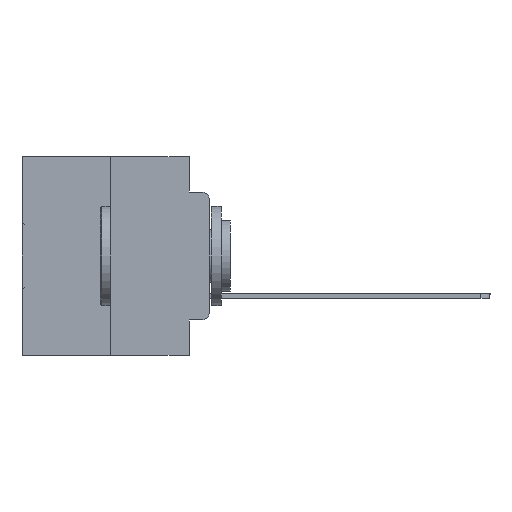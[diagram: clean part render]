
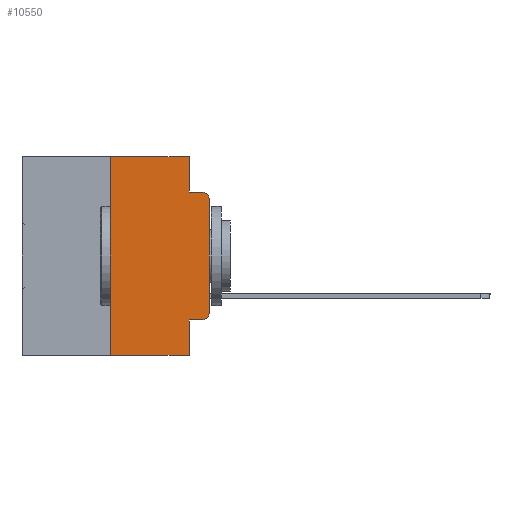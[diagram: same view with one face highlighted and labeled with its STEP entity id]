
A CAD part, left-side view. The second image highlights one B-rep face of the part: STEP entity #10550.
In plain terms, the highlighted planar face has unit normal (-1, 0, 0).
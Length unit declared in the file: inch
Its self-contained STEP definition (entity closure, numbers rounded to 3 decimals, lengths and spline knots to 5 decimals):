
#16 = ORIENTED_EDGE ( 'NONE', *, *, #12953, .T. ) ;
#106 = CARTESIAN_POINT ( 'NONE',  ( 0., 0.051, -0.4115 ) ) ;
#396 = CIRCLE ( 'NONE', #18454, 0.02 ) ;
#503 = CARTESIAN_POINT ( 'NONE',  ( 0., 0.25, 0. ) ) ;
#875 = PLANE ( 'NONE',  #8040 ) ;
#1307 = CARTESIAN_POINT ( 'NONE',  ( 0., 0.02, -0.3915 ) ) ;
#1934 = VECTOR ( 'NONE', #31414, 39.37008 ) ;
#2017 = CARTESIAN_POINT ( 'NONE',  ( 0., 0., -0.3915 ) ) ;
#2045 = DIRECTION ( 'NONE',  ( 0., -1., 0. ) ) ;
#3313 = VERTEX_POINT ( 'NONE', #2017 ) ;
#4301 = LINE ( 'NONE', #26386, #26181 ) ;
#4407 = EDGE_LOOP ( 'NONE', ( #9631, #14332, #9688, #22419, #19656, #26103, #17571, #27976, #16, #5335 ) ) ;
#4494 = VECTOR ( 'NONE', #8327, 39.37008 ) ;
#5335 = ORIENTED_EDGE ( 'NONE', *, *, #7993, .T. ) ;
#6140 = CARTESIAN_POINT ( 'NONE',  ( 0., 0.051, -0.5 ) ) ;
#6204 = CIRCLE ( 'NONE', #24243, 0.02 ) ;
#6547 = CARTESIAN_POINT ( 'NONE',  ( 0., 0.473, 0. ) ) ;
#6802 = VERTEX_POINT ( 'NONE', #503 ) ;
#6828 = CARTESIAN_POINT ( 'NONE',  ( 0., 0.25, -0.5 ) ) ;
#6910 = LINE ( 'NONE', #16754, #1934 ) ;
#7903 = VERTEX_POINT ( 'NONE', #20375 ) ;
#7993 = EDGE_CURVE ( 'NONE', #28216, #3313, #6204, .T. ) ;
#8040 = AXIS2_PLACEMENT_3D ( 'NONE', #6547, #10747, #25894 ) ;
#8327 = DIRECTION ( 'NONE',  ( 0., 0., -1. ) ) ;
#8391 = EDGE_CURVE ( 'NONE', #3313, #31303, #8553, .T. ) ;
#8553 = LINE ( 'NONE', #23393, #24918 ) ;
#8891 = CARTESIAN_POINT ( 'NONE',  ( 0., 0.051, -0.0885 ) ) ;
#9021 = EDGE_CURVE ( 'NONE', #6802, #14356, #26400, .T. ) ;
#9327 = CARTESIAN_POINT ( 'NONE',  ( 0., 0.473, 0. ) ) ;
#9511 = CARTESIAN_POINT ( 'NONE',  ( 0., 0.02, -0.1085 ) ) ;
#9631 = ORIENTED_EDGE ( 'NONE', *, *, #8391, .T. ) ;
#9688 = ORIENTED_EDGE ( 'NONE', *, *, #21601, .F. ) ;
#10180 = EDGE_CURVE ( 'NONE', #21341, #6802, #6910, .T. ) ;
#10550 = ADVANCED_FACE ( 'NONE', ( #16075 ), #875, .F. ) ;
#10659 = DIRECTION ( 'NONE',  ( 0., -1., 0. ) ) ;
#10747 = DIRECTION ( 'NONE',  ( 1., 0., 0. ) ) ;
#11311 = LINE ( 'NONE', #8891, #13076 ) ;
#11527 = VERTEX_POINT ( 'NONE', #23313 ) ;
#11667 = DIRECTION ( 'NONE',  ( -1., 0., 0. ) ) ;
#11932 = CARTESIAN_POINT ( 'NONE',  ( 0., 0.051, 0. ) ) ;
#12953 = EDGE_CURVE ( 'NONE', #11527, #28216, #21914, .T. ) ;
#13076 = VECTOR ( 'NONE', #10659, 39.37008 ) ;
#14150 = CARTESIAN_POINT ( 'NONE',  ( 0., 0.02, -0.4115 ) ) ;
#14224 = EDGE_CURVE ( 'NONE', #31303, #25924, #396, .T. ) ;
#14332 = ORIENTED_EDGE ( 'NONE', *, *, #14224, .T. ) ;
#14356 = VERTEX_POINT ( 'NONE', #11932 ) ;
#14656 = EDGE_CURVE ( 'NONE', #11527, #17836, #4301, .T. ) ;
#14661 = DIRECTION ( 'NONE',  ( -1., 0., 0. ) ) ;
#16075 = FACE_OUTER_BOUND ( 'NONE', #4407, .T. ) ;
#16570 = DIRECTION ( 'NONE',  ( 0., 0., -1. ) ) ;
#16754 = CARTESIAN_POINT ( 'NONE',  ( 0., 0.25, 0. ) ) ;
#17571 = ORIENTED_EDGE ( 'NONE', *, *, #18929, .T. ) ;
#17836 = VERTEX_POINT ( 'NONE', #6140 ) ;
#18389 = DIRECTION ( 'NONE',  ( 0., 0., 1. ) ) ;
#18454 = AXIS2_PLACEMENT_3D ( 'NONE', #9511, #14661, #29141 ) ;
#18929 = EDGE_CURVE ( 'NONE', #21341, #17836, #31671, .T. ) ;
#19203 = VECTOR ( 'NONE', #29694, 39.37008 ) ;
#19656 = ORIENTED_EDGE ( 'NONE', *, *, #9021, .F. ) ;
#20375 = CARTESIAN_POINT ( 'NONE',  ( 0., 0.051, -0.0885 ) ) ;
#20683 = CARTESIAN_POINT ( 'NONE',  ( 0., 0., -0.1085 ) ) ;
#21341 = VERTEX_POINT ( 'NONE', #6828 ) ;
#21601 = EDGE_CURVE ( 'NONE', #7903, #25924, #11311, .T. ) ;
#21914 = LINE ( 'NONE', #106, #24609 ) ;
#22419 = ORIENTED_EDGE ( 'NONE', *, *, #23713, .F. ) ;
#22790 = CARTESIAN_POINT ( 'NONE',  ( 0., 0.473, -0.5 ) ) ;
#23313 = CARTESIAN_POINT ( 'NONE',  ( 0., 0.051, -0.4115 ) ) ;
#23393 = CARTESIAN_POINT ( 'NONE',  ( 0., 0., 0. ) ) ;
#23713 = EDGE_CURVE ( 'NONE', #14356, #7903, #30408, .T. ) ;
#24243 = AXIS2_PLACEMENT_3D ( 'NONE', #1307, #11667, #28563 ) ;
#24479 = DIRECTION ( 'NONE',  ( 0., -1., 0. ) ) ;
#24609 = VECTOR ( 'NONE', #24479, 39.37008 ) ;
#24918 = VECTOR ( 'NONE', #18389, 39.37008 ) ;
#25894 = DIRECTION ( 'NONE',  ( 0., 0., -1. ) ) ;
#25924 = VERTEX_POINT ( 'NONE', #29396 ) ;
#26103 = ORIENTED_EDGE ( 'NONE', *, *, #10180, .F. ) ;
#26181 = VECTOR ( 'NONE', #16570, 39.37008 ) ;
#26386 = CARTESIAN_POINT ( 'NONE',  ( 0., 0.051, 0. ) ) ;
#26400 = LINE ( 'NONE', #9327, #31164 ) ;
#27976 = ORIENTED_EDGE ( 'NONE', *, *, #14656, .F. ) ;
#28216 = VERTEX_POINT ( 'NONE', #14150 ) ;
#28563 = DIRECTION ( 'NONE',  ( 0., 0., -1. ) ) ;
#29141 = DIRECTION ( 'NONE',  ( 0., 0., -1. ) ) ;
#29396 = CARTESIAN_POINT ( 'NONE',  ( 0., 0.02, -0.0885 ) ) ;
#29694 = DIRECTION ( 'NONE',  ( 0., -1., 0. ) ) ;
#30242 = CARTESIAN_POINT ( 'NONE',  ( 0., 0.051, 0. ) ) ;
#30408 = LINE ( 'NONE', #30242, #4494 ) ;
#31164 = VECTOR ( 'NONE', #2045, 39.37008 ) ;
#31303 = VERTEX_POINT ( 'NONE', #20683 ) ;
#31414 = DIRECTION ( 'NONE',  ( 0., 0., 1. ) ) ;
#31671 = LINE ( 'NONE', #22790, #19203 ) ;
